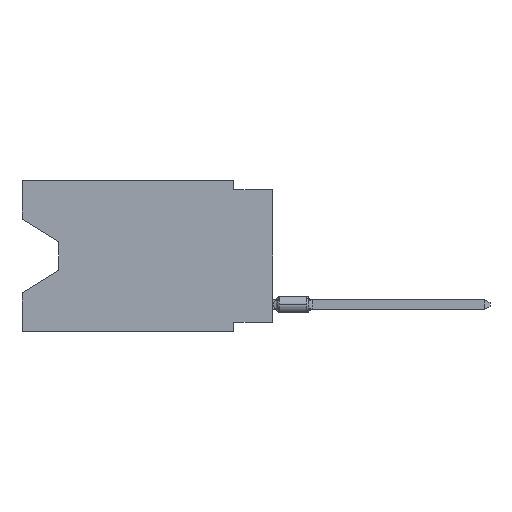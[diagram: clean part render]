
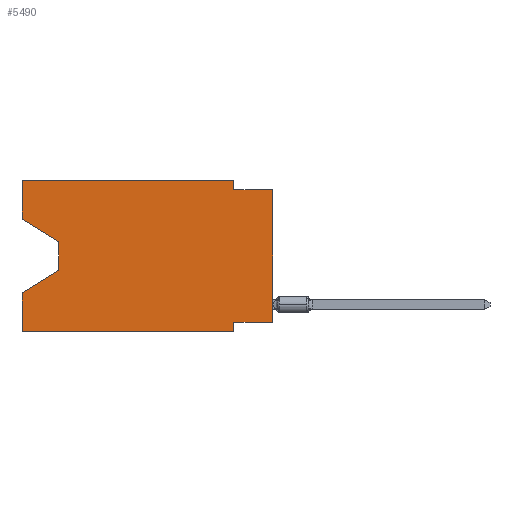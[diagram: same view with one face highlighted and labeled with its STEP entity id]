
A CAD part, left-side view. The second image highlights one B-rep face of the part: STEP entity #5490.
In plain terms, the highlighted planar face has unit normal (-1, 0, 0).
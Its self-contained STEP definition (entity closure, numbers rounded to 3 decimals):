
#274 = VECTOR ( 'NONE', #13403, 1000. ) ;
#377 = LINE ( 'NONE', #17870, #10875 ) ;
#654 = CARTESIAN_POINT ( 'NONE',  ( 0., 16.383, 0. ) ) ;
#662 = LINE ( 'NONE', #15206, #274 ) ;
#874 = ORIENTED_EDGE ( 'NONE', *, *, #11722, .F. ) ;
#884 = CARTESIAN_POINT ( 'NONE',  ( 0., 0., -9.271 ) ) ;
#969 = VERTEX_POINT ( 'NONE', #20712 ) ;
#1187 = VECTOR ( 'NONE', #5002, 1000. ) ;
#1291 = LINE ( 'NONE', #19459, #15659 ) ;
#1529 = DIRECTION ( 'NONE',  ( 0., -0.855, -0.519 ) ) ;
#1569 = DIRECTION ( 'NONE',  ( 0., 0.855, -0.519 ) ) ;
#1827 = EDGE_LOOP ( 'NONE', ( #8907, #16997, #23108, #20266, #4213, #11798, #21838, #19537, #21595, #874, #9028, #10789 ) ) ;
#2352 = EDGE_CURVE ( 'NONE', #4398, #14003, #18149, .T. ) ;
#2377 = CARTESIAN_POINT ( 'NONE',  ( 0., 16.383, 0. ) ) ;
#3067 = DIRECTION ( 'NONE',  ( 0., 0., 1. ) ) ;
#3776 = DIRECTION ( 'NONE',  ( 0., 0., -1. ) ) ;
#3987 = LINE ( 'NONE', #5666, #10650 ) ;
#4213 = ORIENTED_EDGE ( 'NONE', *, *, #12247, .T. ) ;
#4398 = VERTEX_POINT ( 'NONE', #13869 ) ;
#5002 = DIRECTION ( 'NONE',  ( 0., 0., 1. ) ) ;
#5119 = EDGE_CURVE ( 'NONE', #12377, #16296, #22676, .T. ) ;
#5490 = ADVANCED_FACE ( 'NONE', ( #13510 ), #19163, .F. ) ;
#5591 = EDGE_CURVE ( 'NONE', #19889, #12377, #11932, .T. ) ;
#5666 = CARTESIAN_POINT ( 'NONE',  ( 0., 16.383, -9.906 ) ) ;
#6382 = CARTESIAN_POINT ( 'NONE',  ( 0., 2.54, -9.906 ) ) ;
#6719 = VECTOR ( 'NONE', #15671, 1000. ) ;
#7409 = DIRECTION ( 'NONE',  ( 0., -1., 0. ) ) ;
#7652 = CARTESIAN_POINT ( 'NONE',  ( 0., 13.97, -4.013 ) ) ;
#7996 = EDGE_CURVE ( 'NONE', #19889, #12729, #19555, .T. ) ;
#8688 = CARTESIAN_POINT ( 'NONE',  ( 0., 16.383, -9.906 ) ) ;
#8736 = DIRECTION ( 'NONE',  ( 0., 0., 1. ) ) ;
#8787 = EDGE_CURVE ( 'NONE', #22496, #18274, #14387, .T. ) ;
#8907 = ORIENTED_EDGE ( 'NONE', *, *, #12701, .T. ) ;
#9028 = ORIENTED_EDGE ( 'NONE', *, *, #14181, .F. ) ;
#9940 = CARTESIAN_POINT ( 'NONE',  ( 0., 16.383, 0. ) ) ;
#10565 = VERTEX_POINT ( 'NONE', #17129 ) ;
#10650 = VECTOR ( 'NONE', #18919, 1000. ) ;
#10789 = ORIENTED_EDGE ( 'NONE', *, *, #8787, .F. ) ;
#10875 = VECTOR ( 'NONE', #12442, 1000. ) ;
#11722 = EDGE_CURVE ( 'NONE', #10565, #969, #662, .T. ) ;
#11798 = ORIENTED_EDGE ( 'NONE', *, *, #5119, .F. ) ;
#11932 = LINE ( 'NONE', #884, #6719 ) ;
#12014 = VERTEX_POINT ( 'NONE', #8688 ) ;
#12247 = EDGE_CURVE ( 'NONE', #12014, #16296, #3987, .T. ) ;
#12377 = VERTEX_POINT ( 'NONE', #19165 ) ;
#12442 = DIRECTION ( 'NONE',  ( 0., 0., -1. ) ) ;
#12701 = EDGE_CURVE ( 'NONE', #22496, #20056, #1291, .T. ) ;
#12729 = VERTEX_POINT ( 'NONE', #23415 ) ;
#12927 = CARTESIAN_POINT ( 'NONE',  ( 0., 2.54, -9.906 ) ) ;
#13149 = CARTESIAN_POINT ( 'NONE',  ( 0., 16.383, -2.546 ) ) ;
#13403 = DIRECTION ( 'NONE',  ( 0., 0., -1. ) ) ;
#13510 = FACE_OUTER_BOUND ( 'NONE', #1827, .T. ) ;
#13858 = VECTOR ( 'NONE', #7409, 1000. ) ;
#13869 = CARTESIAN_POINT ( 'NONE',  ( 0., 13.97, -5.893 ) ) ;
#14003 = VERTEX_POINT ( 'NONE', #20948 ) ;
#14181 = EDGE_CURVE ( 'NONE', #18274, #10565, #20397, .T. ) ;
#14264 = CARTESIAN_POINT ( 'NONE',  ( 0., 16.383, 0. ) ) ;
#14293 = CARTESIAN_POINT ( 'NONE',  ( 0., 0., -9.271 ) ) ;
#14387 = LINE ( 'NONE', #14264, #18550 ) ;
#14406 = EDGE_CURVE ( 'NONE', #20056, #4398, #377, .T. ) ;
#15089 = VECTOR ( 'NONE', #22445, 1000. ) ;
#15206 = CARTESIAN_POINT ( 'NONE',  ( 0., 2.54, 0. ) ) ;
#15425 = DIRECTION ( 'NONE',  ( 1., 0., 0. ) ) ;
#15659 = VECTOR ( 'NONE', #1529, 1000. ) ;
#15671 = DIRECTION ( 'NONE',  ( 0., 1., 0. ) ) ;
#15954 = VECTOR ( 'NONE', #3067, 1000. ) ;
#15992 = LINE ( 'NONE', #19367, #1187 ) ;
#16296 = VERTEX_POINT ( 'NONE', #6382 ) ;
#16344 = LINE ( 'NONE', #23673, #13858 ) ;
#16356 = CARTESIAN_POINT ( 'NONE',  ( 0., 13.97, -5.893 ) ) ;
#16997 = ORIENTED_EDGE ( 'NONE', *, *, #14406, .T. ) ;
#17129 = CARTESIAN_POINT ( 'NONE',  ( 0., 2.54, 0. ) ) ;
#17870 = CARTESIAN_POINT ( 'NONE',  ( 0., 13.97, -4.013 ) ) ;
#18149 = LINE ( 'NONE', #16356, #19061 ) ;
#18274 = VERTEX_POINT ( 'NONE', #2377 ) ;
#18550 = VECTOR ( 'NONE', #8736, 1000. ) ;
#18919 = DIRECTION ( 'NONE',  ( 0., -1., 0. ) ) ;
#19061 = VECTOR ( 'NONE', #1569, 1000. ) ;
#19163 = PLANE ( 'NONE',  #19408 ) ;
#19165 = CARTESIAN_POINT ( 'NONE',  ( 0., 2.54, -9.271 ) ) ;
#19367 = CARTESIAN_POINT ( 'NONE',  ( 0., 16.383, 0. ) ) ;
#19408 = AXIS2_PLACEMENT_3D ( 'NONE', #654, #15425, #22653 ) ;
#19459 = CARTESIAN_POINT ( 'NONE',  ( 0., 16.383, -2.546 ) ) ;
#19537 = ORIENTED_EDGE ( 'NONE', *, *, #7996, .T. ) ;
#19555 = LINE ( 'NONE', #19669, #15954 ) ;
#19669 = CARTESIAN_POINT ( 'NONE',  ( 0., 0., 0. ) ) ;
#19761 = EDGE_CURVE ( 'NONE', #12014, #14003, #15992, .T. ) ;
#19889 = VERTEX_POINT ( 'NONE', #14293 ) ;
#19984 = EDGE_CURVE ( 'NONE', #969, #12729, #16344, .T. ) ;
#20056 = VERTEX_POINT ( 'NONE', #7652 ) ;
#20266 = ORIENTED_EDGE ( 'NONE', *, *, #19761, .F. ) ;
#20397 = LINE ( 'NONE', #9940, #15089 ) ;
#20712 = CARTESIAN_POINT ( 'NONE',  ( 0., 2.54, -0.635 ) ) ;
#20948 = CARTESIAN_POINT ( 'NONE',  ( 0., 16.383, -7.36 ) ) ;
#21595 = ORIENTED_EDGE ( 'NONE', *, *, #19984, .F. ) ;
#21838 = ORIENTED_EDGE ( 'NONE', *, *, #5591, .F. ) ;
#22445 = DIRECTION ( 'NONE',  ( 0., -1., 0. ) ) ;
#22496 = VERTEX_POINT ( 'NONE', #13149 ) ;
#22653 = DIRECTION ( 'NONE',  ( 0., 0., -1. ) ) ;
#22676 = LINE ( 'NONE', #12927, #23222 ) ;
#23108 = ORIENTED_EDGE ( 'NONE', *, *, #2352, .T. ) ;
#23222 = VECTOR ( 'NONE', #3776, 1000. ) ;
#23415 = CARTESIAN_POINT ( 'NONE',  ( 0., 0., -0.635 ) ) ;
#23673 = CARTESIAN_POINT ( 'NONE',  ( 0., 0., -0.635 ) ) ;
